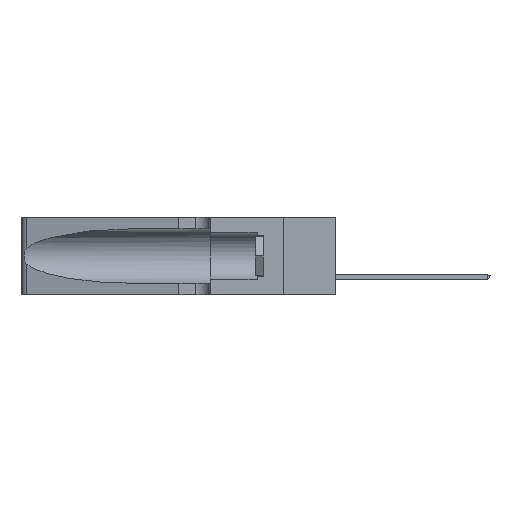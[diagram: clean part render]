
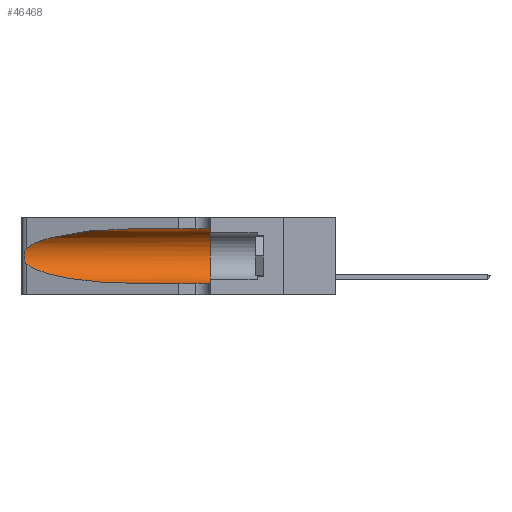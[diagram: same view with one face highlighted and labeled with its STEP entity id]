
A CAD part, left-side view. The second image highlights one B-rep face of the part: STEP entity #46468.
In plain terms, the highlighted cylindrical face has radius 3.308 mm (diameter 6.617 mm), a partial arc.
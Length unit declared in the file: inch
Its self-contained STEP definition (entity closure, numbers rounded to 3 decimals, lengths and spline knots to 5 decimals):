
#360 = EDGE_CURVE ( 'NONE', #43586, #21909, #18567, .T. ) ;
#2202 = AXIS2_PLACEMENT_3D ( 'NONE', #48493, #36728, #28962 ) ;
#2675 = VERTEX_POINT ( 'NONE', #45024 ) ;
#3668 = LINE ( 'NONE', #46616, #15904 ) ;
#5435 = EDGE_CURVE ( 'NONE', #8979, #18592, #22993, .T. ) ;
#5544 = CARTESIAN_POINT ( 'NONE',  ( 0.26017, 1.23833, 0.17102 ) ) ;
#6224 = CIRCLE ( 'NONE', #2202, 0.13025 ) ;
#6679 = CARTESIAN_POINT ( 'NONE',  ( 0.2373, 1.15595, 0.28018 ) ) ;
#7448 = CARTESIAN_POINT ( 'NONE',  ( 0.25555, 1.22994, 0.2215 ) ) ;
#8670 = ORIENTED_EDGE ( 'NONE', *, *, #31209, .T. ) ;
#8698 = FACE_OUTER_BOUND ( 'NONE', #14220, .T. ) ;
#8979 = VERTEX_POINT ( 'NONE', #23129 ) ;
#9584 = CARTESIAN_POINT ( 'NONE',  ( 0.1305, 0.72297, 0.05475 ) ) ;
#10018 = CARTESIAN_POINT ( 'NONE',  ( 0.25555, 1.22993, 0.14849 ) ) ;
#10214 = CARTESIAN_POINT ( 'NONE',  ( 0.26075, 1.23896, 0.178 ) ) ;
#12767 = DIRECTION ( 'NONE',  ( 0., -1., 0. ) ) ;
#13379 = EDGE_CURVE ( 'NONE', #18592, #43586, #37443, .T. ) ;
#13800 = CARTESIAN_POINT ( 'NONE',  ( 0.25856, 1.23593, 0.16098 ) ) ;
#13986 = CARTESIAN_POINT ( 'NONE',  ( 0.25789, 1.23486, 0.15765 ) ) ;
#14162 = CARTESIAN_POINT ( 'NONE',  ( 0.25639, 1.23186, 0.15144 ) ) ;
#14220 = EDGE_LOOP ( 'NONE', ( #8670, #15361, #40076, #27390, #50293, #14865 ) ) ;
#14865 = ORIENTED_EDGE ( 'NONE', *, *, #33558, .F. ) ;
#14946 = CARTESIAN_POINT ( 'NONE',  ( 0.25487, 1.22718, 0.22369 ) ) ;
#15361 = ORIENTED_EDGE ( 'NONE', *, *, #5435, .T. ) ;
#15904 = VECTOR ( 'NONE', #50765, 39.37008 ) ;
#18567 = LINE ( 'NONE', #47930, #19152 ) ;
#18592 = VERTEX_POINT ( 'NONE', #41717 ) ;
#18735 = DIRECTION ( 'NONE',  ( 0., 0., -1. ) ) ;
#19152 = VECTOR ( 'NONE', #12767, 39.37008 ) ;
#19216 =( BOUNDED_CURVE ( )  B_SPLINE_CURVE ( 3, ( #45425, #30061, #6679, #21912 ),
 .UNSPECIFIED., .F., .T. ) 
 B_SPLINE_CURVE_WITH_KNOTS ( ( 4, 4 ),
 ( 1.5708, 2.84003 ),
 .UNSPECIFIED. ) 
 CURVE ( )  GEOMETRIC_REPRESENTATION_ITEM ( )  RATIONAL_B_SPLINE_CURVE ( ( 1., 0.87, 0.87, 1. ) ) 
 REPRESENTATION_ITEM ( '' )  );
#19874 = CARTESIAN_POINT ( 'NONE',  ( 0.26018, 1.23835, 0.19895 ) ) ;
#21485 = CARTESIAN_POINT ( 'NONE',  ( 0.2373, 1.15595, 0.08982 ) ) ;
#21909 = VERTEX_POINT ( 'NONE', #26571 ) ;
#21912 = CARTESIAN_POINT ( 'NONE',  ( 0.25487, 1.22718, 0.22369 ) ) ;
#22850 = CARTESIAN_POINT ( 'NONE',  ( 0.25787, 1.23484, 0.2124 ) ) ;
#22951 = CYLINDRICAL_SURFACE ( 'NONE', #34181, 0.13025 ) ;
#22993 = B_SPLINE_CURVE_WITH_KNOTS ( 'NONE', 3,
 ( #14946, #7448, #46542, #22850, #27027, #19874, #47499, #10214, #5544, #13800, #13986, #14162, #10018, #41681 ),
 .UNSPECIFIED., .F., .F.,
 ( 4, 2, 2, 2, 2, 2, 4 ),
 ( 0., 0.00027, 0.00053, 0.00107, 0.0016, 0.00187, 0.00214 ),
 .UNSPECIFIED. ) ;
#23129 = CARTESIAN_POINT ( 'NONE',  ( 0.25487, 1.22718, 0.22369 ) ) ;
#26571 = CARTESIAN_POINT ( 'NONE',  ( 0.1305, 0.35, 0.05475 ) ) ;
#27027 = CARTESIAN_POINT ( 'NONE',  ( 0.25854, 1.2359, 0.20912 ) ) ;
#27390 = ORIENTED_EDGE ( 'NONE', *, *, #360, .T. ) ;
#28962 = DIRECTION ( 'NONE',  ( 0., 0., 1. ) ) ;
#30061 = CARTESIAN_POINT ( 'NONE',  ( 0.18966, 0.96281, 0.31525 ) ) ;
#31209 = EDGE_CURVE ( 'NONE', #2675, #8979, #19216, .T. ) ;
#33558 = EDGE_CURVE ( 'NONE', #2675, #39719, #3668, .T. ) ;
#34181 = AXIS2_PLACEMENT_3D ( 'NONE', #45847, #38539, #18735 ) ;
#36728 = DIRECTION ( 'NONE',  ( 0., 1., 0. ) ) ;
#37443 =( BOUNDED_CURVE ( )  B_SPLINE_CURVE ( 3, ( #45009, #21485, #41651, #9584 ),
 .UNSPECIFIED., .F., .F. ) 
 B_SPLINE_CURVE_WITH_KNOTS ( ( 4, 4 ),
 ( 3.44316, 4.71239 ),
 .UNSPECIFIED. ) 
 CURVE ( )  GEOMETRIC_REPRESENTATION_ITEM ( )  RATIONAL_B_SPLINE_CURVE ( ( 1., 0.87, 0.87, 1. ) ) 
 REPRESENTATION_ITEM ( '' )  );
#37531 = CARTESIAN_POINT ( 'NONE',  ( 0.1305, 0.35, 0.31525 ) ) ;
#38539 = DIRECTION ( 'NONE',  ( 0., -1., 0. ) ) ;
#39719 = VERTEX_POINT ( 'NONE', #37531 ) ;
#40076 = ORIENTED_EDGE ( 'NONE', *, *, #13379, .T. ) ;
#41651 = CARTESIAN_POINT ( 'NONE',  ( 0.18966, 0.96281, 0.05475 ) ) ;
#41681 = CARTESIAN_POINT ( 'NONE',  ( 0.25487, 1.22718, 0.14631 ) ) ;
#41717 = CARTESIAN_POINT ( 'NONE',  ( 0.25487, 1.22718, 0.14631 ) ) ;
#43586 = VERTEX_POINT ( 'NONE', #43733 ) ;
#43733 = CARTESIAN_POINT ( 'NONE',  ( 0.1305, 0.72297, 0.05475 ) ) ;
#45009 = CARTESIAN_POINT ( 'NONE',  ( 0.25487, 1.22718, 0.14631 ) ) ;
#45024 = CARTESIAN_POINT ( 'NONE',  ( 0.1305, 0.72297, 0.31525 ) ) ;
#45425 = CARTESIAN_POINT ( 'NONE',  ( 0.1305, 0.72297, 0.31525 ) ) ;
#45847 = CARTESIAN_POINT ( 'NONE',  ( 0.1305, 1.61858, 0.185 ) ) ;
#46468 = ADVANCED_FACE ( 'NONE', ( #8698 ), #22951, .F. ) ;
#46542 = CARTESIAN_POINT ( 'NONE',  ( 0.25639, 1.23184, 0.21858 ) ) ;
#46616 = CARTESIAN_POINT ( 'NONE',  ( 0.1305, 1.61858, 0.31525 ) ) ;
#47499 = CARTESIAN_POINT ( 'NONE',  ( 0.26075, 1.23896, 0.19203 ) ) ;
#47930 = CARTESIAN_POINT ( 'NONE',  ( 0.1305, 1.61858, 0.05475 ) ) ;
#48493 = CARTESIAN_POINT ( 'NONE',  ( 0.1305, 0.35, 0.185 ) ) ;
#49467 = EDGE_CURVE ( 'NONE', #39719, #21909, #6224, .T. ) ;
#50293 = ORIENTED_EDGE ( 'NONE', *, *, #49467, .F. ) ;
#50765 = DIRECTION ( 'NONE',  ( 0., -1., 0. ) ) ;
